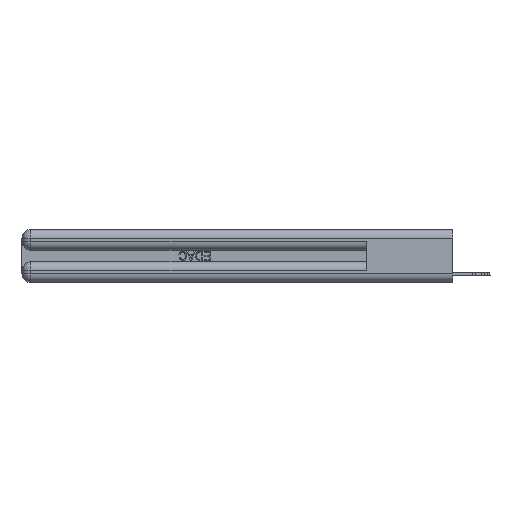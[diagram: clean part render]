
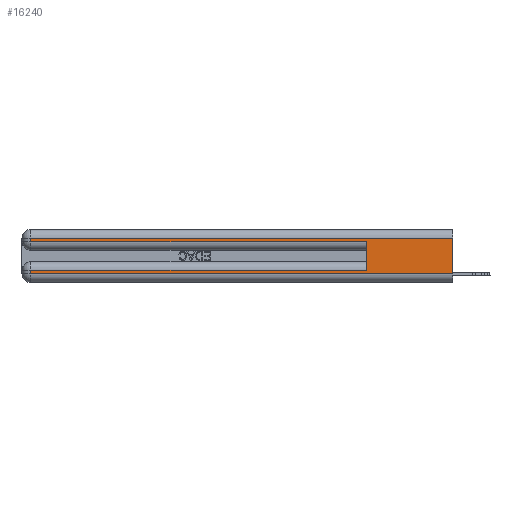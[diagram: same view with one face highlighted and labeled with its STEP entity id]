
A CAD part, left-side view. The second image highlights one B-rep face of the part: STEP entity #16240.
In plain terms, the highlighted planar face has unit normal (-1, 0, 0).
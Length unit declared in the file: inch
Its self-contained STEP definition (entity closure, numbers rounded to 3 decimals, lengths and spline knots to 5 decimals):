
#962 = EDGE_CURVE ( 'NONE', #21425, #13256, #33375, .T. ) ;
#1026 = VERTEX_POINT ( 'NONE', #22559 ) ;
#1550 = DIRECTION ( 'NONE',  ( 0., -1., 0. ) ) ;
#1990 = EDGE_LOOP ( 'NONE', ( #29939, #8372, #3606, #24235, #20360, #13332, #31018, #8158 ) ) ;
#2229 = LINE ( 'NONE', #12871, #14839 ) ;
#2358 = LINE ( 'NONE', #15640, #12057 ) ;
#2511 = DIRECTION ( 'NONE',  ( 0., 1., 0. ) ) ;
#2935 = VERTEX_POINT ( 'NONE', #12686 ) ;
#3606 = ORIENTED_EDGE ( 'NONE', *, *, #21192, .T. ) ;
#3844 = CARTESIAN_POINT ( 'NONE',  ( 0., 0., 0.37 ) ) ;
#4559 = DIRECTION ( 'NONE',  ( 0., 0., -1. ) ) ;
#4655 = CARTESIAN_POINT ( 'NONE',  ( 0., 2.94, 0.085 ) ) ;
#4684 = EDGE_CURVE ( 'NONE', #34493, #17050, #5143, .T. ) ;
#5143 = LINE ( 'NONE', #7045, #32787 ) ;
#5960 = LINE ( 'NONE', #16627, #18972 ) ;
#7031 = CARTESIAN_POINT ( 'NONE',  ( 0., 0., 0.06 ) ) ;
#7045 = CARTESIAN_POINT ( 'NONE',  ( 0., 0., 0.085 ) ) ;
#7174 = LINE ( 'NONE', #30953, #17355 ) ;
#7872 = LINE ( 'NONE', #18577, #21829 ) ;
#8158 = ORIENTED_EDGE ( 'NONE', *, *, #962, .T. ) ;
#8372 = ORIENTED_EDGE ( 'NONE', *, *, #29646, .T. ) ;
#8782 = AXIS2_PLACEMENT_3D ( 'NONE', #10132, #9959, #4559 ) ;
#9223 = VERTEX_POINT ( 'NONE', #24051 ) ;
#9959 = DIRECTION ( 'NONE',  ( 1., 0., 0. ) ) ;
#10132 = CARTESIAN_POINT ( 'NONE',  ( 0., 0., 0.37 ) ) ;
#12057 = VECTOR ( 'NONE', #34496, 39.37008 ) ;
#12390 = EDGE_CURVE ( 'NONE', #34493, #34092, #5960, .T. ) ;
#12686 = CARTESIAN_POINT ( 'NONE',  ( 0., 2.94, 0.285 ) ) ;
#12871 = CARTESIAN_POINT ( 'NONE',  ( 0., 2.94, 0.37 ) ) ;
#13256 = VERTEX_POINT ( 'NONE', #7031 ) ;
#13332 = ORIENTED_EDGE ( 'NONE', *, *, #4684, .T. ) ;
#14839 = VECTOR ( 'NONE', #34209, 39.37008 ) ;
#15640 = CARTESIAN_POINT ( 'NONE',  ( 0., 0., 0.31 ) ) ;
#15905 = DIRECTION ( 'NONE',  ( 0., -1., 0. ) ) ;
#16240 = ADVANCED_FACE ( 'NONE', ( #23089 ), #31130, .F. ) ;
#16627 = CARTESIAN_POINT ( 'NONE',  ( 0., 0.6, 0.145 ) ) ;
#17050 = VERTEX_POINT ( 'NONE', #4655 ) ;
#17355 = VECTOR ( 'NONE', #28158, 39.37008 ) ;
#17810 = LINE ( 'NONE', #3844, #21073 ) ;
#18577 = CARTESIAN_POINT ( 'NONE',  ( 0., 0., 0.285 ) ) ;
#18972 = VECTOR ( 'NONE', #32539, 39.37008 ) ;
#20360 = ORIENTED_EDGE ( 'NONE', *, *, #12390, .F. ) ;
#21073 = VECTOR ( 'NONE', #30252, 39.37008 ) ;
#21192 = EDGE_CURVE ( 'NONE', #9223, #2935, #7174, .T. ) ;
#21305 = EDGE_CURVE ( 'NONE', #2935, #34092, #7872, .T. ) ;
#21425 = VERTEX_POINT ( 'NONE', #27095 ) ;
#21554 = CARTESIAN_POINT ( 'NONE',  ( 0., 0.6, 0.285 ) ) ;
#21829 = VECTOR ( 'NONE', #15905, 39.37008 ) ;
#22559 = CARTESIAN_POINT ( 'NONE',  ( 0., 0., 0.31 ) ) ;
#22571 = CARTESIAN_POINT ( 'NONE',  ( 0., 0.6, 0.085 ) ) ;
#23089 = FACE_OUTER_BOUND ( 'NONE', #1990, .T. ) ;
#24051 = CARTESIAN_POINT ( 'NONE',  ( 0., 2.94, 0.31 ) ) ;
#24235 = ORIENTED_EDGE ( 'NONE', *, *, #21305, .T. ) ;
#27095 = CARTESIAN_POINT ( 'NONE',  ( 0., 2.94, 0.06 ) ) ;
#28158 = DIRECTION ( 'NONE',  ( 0., 0., -1. ) ) ;
#29646 = EDGE_CURVE ( 'NONE', #1026, #9223, #2358, .T. ) ;
#29939 = ORIENTED_EDGE ( 'NONE', *, *, #30296, .F. ) ;
#30069 = CARTESIAN_POINT ( 'NONE',  ( 0., 0., 0.06 ) ) ;
#30252 = DIRECTION ( 'NONE',  ( 0., 0., -1. ) ) ;
#30296 = EDGE_CURVE ( 'NONE', #1026, #13256, #17810, .T. ) ;
#30565 = EDGE_CURVE ( 'NONE', #17050, #21425, #2229, .T. ) ;
#30953 = CARTESIAN_POINT ( 'NONE',  ( 0., 2.94, 0.37 ) ) ;
#31018 = ORIENTED_EDGE ( 'NONE', *, *, #30565, .T. ) ;
#31130 = PLANE ( 'NONE',  #8782 ) ;
#31196 = VECTOR ( 'NONE', #1550, 39.37008 ) ;
#32539 = DIRECTION ( 'NONE',  ( 0., 0., 1. ) ) ;
#32787 = VECTOR ( 'NONE', #2511, 39.37008 ) ;
#33375 = LINE ( 'NONE', #30069, #31196 ) ;
#34092 = VERTEX_POINT ( 'NONE', #21554 ) ;
#34209 = DIRECTION ( 'NONE',  ( 0., 0., -1. ) ) ;
#34493 = VERTEX_POINT ( 'NONE', #22571 ) ;
#34496 = DIRECTION ( 'NONE',  ( 0., 1., 0. ) ) ;
